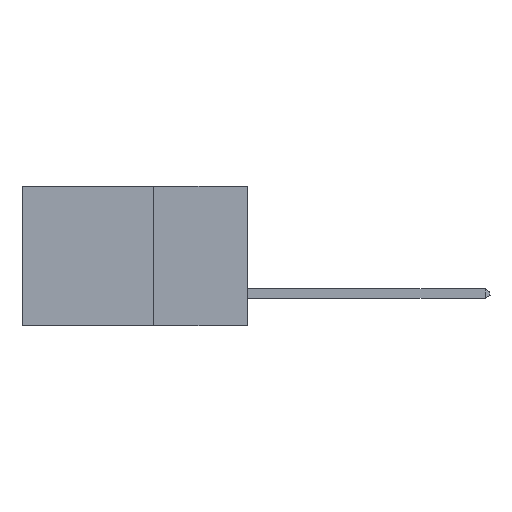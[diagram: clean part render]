
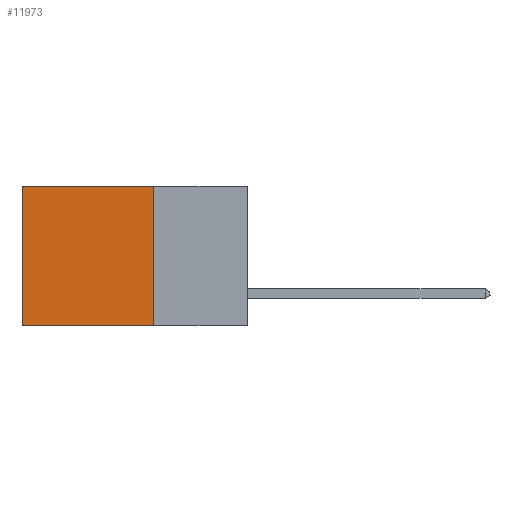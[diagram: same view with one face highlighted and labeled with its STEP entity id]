
A CAD part, left-side view. The second image highlights one B-rep face of the part: STEP entity #11973.
In plain terms, the highlighted planar face has unit normal (-1, 0, 0).
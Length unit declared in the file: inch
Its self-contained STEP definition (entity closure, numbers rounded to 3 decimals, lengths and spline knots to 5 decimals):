
#1116 = VECTOR ( 'NONE', #3633, 39.37008 ) ;
#1358 = FACE_OUTER_BOUND ( 'NONE', #12702, .T. ) ;
#1366 = CARTESIAN_POINT ( 'NONE',  ( 0.298, 0.25, 0. ) ) ;
#1556 = LINE ( 'NONE', #1366, #12306 ) ;
#2472 = VERTEX_POINT ( 'NONE', #9789 ) ;
#2678 = EDGE_CURVE ( 'NONE', #13830, #2472, #9784, .T. ) ;
#2713 = CARTESIAN_POINT ( 'NONE',  ( 0.298, 0.25, 0. ) ) ;
#3524 = EDGE_CURVE ( 'NONE', #2472, #8594, #13096, .T. ) ;
#3633 = DIRECTION ( 'NONE',  ( 0., 0., -1. ) ) ;
#3702 = VERTEX_POINT ( 'NONE', #11444 ) ;
#4006 = DIRECTION ( 'NONE',  ( 0., 0., -1. ) ) ;
#4813 = EDGE_CURVE ( 'NONE', #13830, #3702, #1556, .T. ) ;
#5162 = LINE ( 'NONE', #13354, #1116 ) ;
#6238 = ORIENTED_EDGE ( 'NONE', *, *, #4813, .T. ) ;
#6319 = CARTESIAN_POINT ( 'NONE',  ( 0.298, 0.25, 0. ) ) ;
#6427 = DIRECTION ( 'NONE',  ( 0., 1., 0. ) ) ;
#7862 = CARTESIAN_POINT ( 'NONE',  ( 0.298, 0.25, 0. ) ) ;
#8594 = VERTEX_POINT ( 'NONE', #14347 ) ;
#8958 = PLANE ( 'NONE',  #11101 ) ;
#9522 = ORIENTED_EDGE ( 'NONE', *, *, #3524, .F. ) ;
#9784 = LINE ( 'NONE', #6319, #11879 ) ;
#9789 = CARTESIAN_POINT ( 'NONE',  ( 0.298, 0.25, -0.37 ) ) ;
#9837 = ORIENTED_EDGE ( 'NONE', *, *, #2678, .F. ) ;
#11101 = AXIS2_PLACEMENT_3D ( 'NONE', #2713, #13879, #4006 ) ;
#11444 = CARTESIAN_POINT ( 'NONE',  ( 0.298, 0.6, 0. ) ) ;
#11879 = VECTOR ( 'NONE', #13497, 39.37008 ) ;
#11973 = ADVANCED_FACE ( 'NONE', ( #1358 ), #8958, .F. ) ;
#12306 = VECTOR ( 'NONE', #14979, 39.37008 ) ;
#12638 = CARTESIAN_POINT ( 'NONE',  ( 0.298, 0.25, -0.37 ) ) ;
#12702 = EDGE_LOOP ( 'NONE', ( #15006, #9522, #9837, #6238 ) ) ;
#13096 = LINE ( 'NONE', #12638, #14433 ) ;
#13123 = EDGE_CURVE ( 'NONE', #3702, #8594, #5162, .T. ) ;
#13354 = CARTESIAN_POINT ( 'NONE',  ( 0.298, 0.6, 0. ) ) ;
#13497 = DIRECTION ( 'NONE',  ( 0., 0., -1. ) ) ;
#13830 = VERTEX_POINT ( 'NONE', #7862 ) ;
#13879 = DIRECTION ( 'NONE',  ( 1., 0., 0. ) ) ;
#14347 = CARTESIAN_POINT ( 'NONE',  ( 0.298, 0.6, -0.37 ) ) ;
#14433 = VECTOR ( 'NONE', #6427, 39.37008 ) ;
#14979 = DIRECTION ( 'NONE',  ( 0., 1., 0. ) ) ;
#15006 = ORIENTED_EDGE ( 'NONE', *, *, #13123, .T. ) ;
